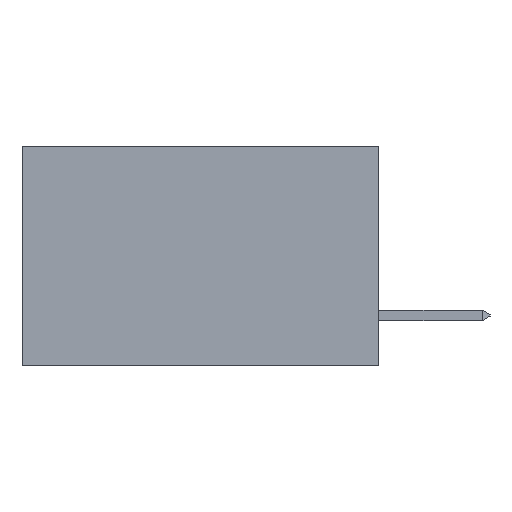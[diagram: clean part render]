
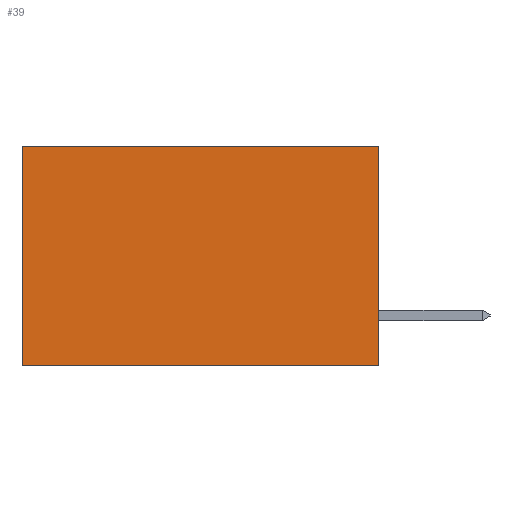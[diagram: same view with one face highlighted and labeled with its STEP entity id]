
A CAD part, left-side view. The second image highlights one B-rep face of the part: STEP entity #39.
In plain terms, the highlighted planar face has unit normal (-1, 0, 0).
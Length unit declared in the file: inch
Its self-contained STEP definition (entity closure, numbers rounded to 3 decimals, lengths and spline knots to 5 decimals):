
#39 = ADVANCED_FACE ( 'NONE', ( #3244 ), #16205, .F. ) ;
#1016 = VECTOR ( 'NONE', #17708, 39.37008 ) ;
#1795 = CARTESIAN_POINT ( 'NONE',  ( 0.2615, 0., -0.37 ) ) ;
#2715 = CARTESIAN_POINT ( 'NONE',  ( 0.2615, 0., 0. ) ) ;
#2797 = CARTESIAN_POINT ( 'NONE',  ( 0.2615, 0., -0.37 ) ) ;
#2829 = DIRECTION ( 'NONE',  ( 0., 0., -1. ) ) ;
#2939 = VECTOR ( 'NONE', #2829, 39.37008 ) ;
#3064 = ORIENTED_EDGE ( 'NONE', *, *, #10670, .F. ) ;
#3244 = FACE_OUTER_BOUND ( 'NONE', #5483, .T. ) ;
#3481 = LINE ( 'NONE', #15144, #10485 ) ;
#3550 = ORIENTED_EDGE ( 'NONE', *, *, #14056, .F. ) ;
#4645 = AXIS2_PLACEMENT_3D ( 'NONE', #2797, #12170, #14245 ) ;
#5473 = CARTESIAN_POINT ( 'NONE',  ( 0.2615, 0.6, 0. ) ) ;
#5483 = EDGE_LOOP ( 'NONE', ( #14730, #3550, #3064, #7090 ) ) ;
#5993 = VERTEX_POINT ( 'NONE', #7774 ) ;
#7090 = ORIENTED_EDGE ( 'NONE', *, *, #9455, .T. ) ;
#7151 = CARTESIAN_POINT ( 'NONE',  ( 0.2615, 0.6, -0.37 ) ) ;
#7230 = CARTESIAN_POINT ( 'NONE',  ( 0.2615, 0.6, -0.37 ) ) ;
#7774 = CARTESIAN_POINT ( 'NONE',  ( 0.2615, 0., -0.37 ) ) ;
#9455 = EDGE_CURVE ( 'NONE', #14869, #9603, #12067, .T. ) ;
#9603 = VERTEX_POINT ( 'NONE', #5473 ) ;
#9736 = LINE ( 'NONE', #1795, #13440 ) ;
#10359 = DIRECTION ( 'NONE',  ( 0., 0., -1. ) ) ;
#10485 = VECTOR ( 'NONE', #17791, 39.37008 ) ;
#10670 = EDGE_CURVE ( 'NONE', #14869, #5993, #9736, .T. ) ;
#12067 = LINE ( 'NONE', #15001, #1016 ) ;
#12170 = DIRECTION ( 'NONE',  ( 1., 0., 0. ) ) ;
#13440 = VECTOR ( 'NONE', #10359, 39.37008 ) ;
#14056 = EDGE_CURVE ( 'NONE', #5993, #17947, #3481, .T. ) ;
#14157 = LINE ( 'NONE', #7151, #2939 ) ;
#14245 = DIRECTION ( 'NONE',  ( 0., 0., -1. ) ) ;
#14730 = ORIENTED_EDGE ( 'NONE', *, *, #15561, .T. ) ;
#14869 = VERTEX_POINT ( 'NONE', #2715 ) ;
#15001 = CARTESIAN_POINT ( 'NONE',  ( 0.2615, 0., 0. ) ) ;
#15144 = CARTESIAN_POINT ( 'NONE',  ( 0.2615, 0., -0.37 ) ) ;
#15561 = EDGE_CURVE ( 'NONE', #9603, #17947, #14157, .T. ) ;
#16205 = PLANE ( 'NONE',  #4645 ) ;
#17708 = DIRECTION ( 'NONE',  ( 0., 1., 0. ) ) ;
#17791 = DIRECTION ( 'NONE',  ( 0., 1., 0. ) ) ;
#17947 = VERTEX_POINT ( 'NONE', #7230 ) ;
